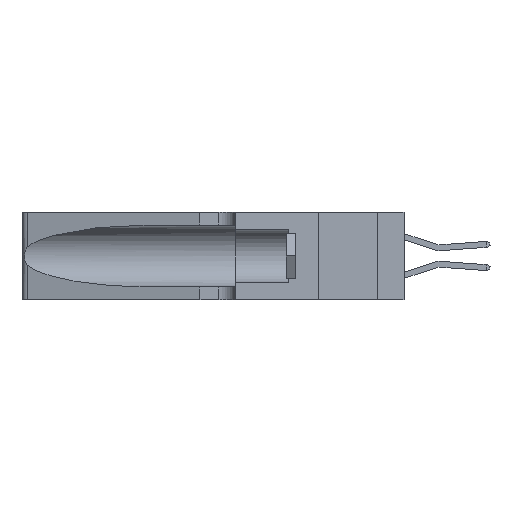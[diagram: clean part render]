
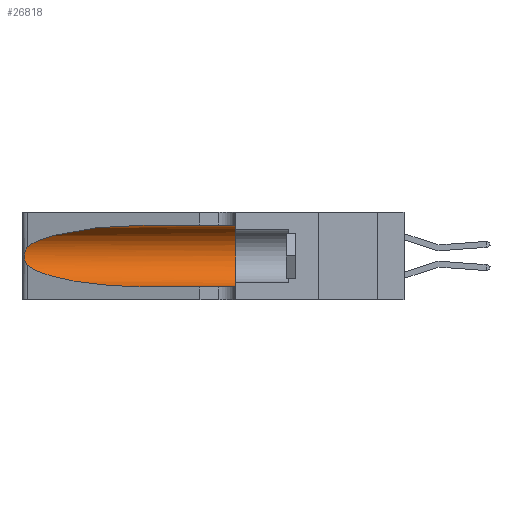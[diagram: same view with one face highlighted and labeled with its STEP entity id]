
A CAD part, left-side view. The second image highlights one B-rep face of the part: STEP entity #26818.
In plain terms, the highlighted cylindrical face has radius 3.308 mm (diameter 6.617 mm), a partial arc.
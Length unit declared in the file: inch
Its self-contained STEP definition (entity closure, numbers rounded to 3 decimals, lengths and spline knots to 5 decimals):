
#144 = CARTESIAN_POINT ( 'NONE',  ( 0.25856, 1.23593, 0.16098 ) ) ;
#509 = CIRCLE ( 'NONE', #16117, 0.13025 ) ;
#758 = CARTESIAN_POINT ( 'NONE',  ( 0.1305, 1.61858, 0.05475 ) ) ;
#2188 = EDGE_CURVE ( 'NONE', #5436, #7439, #509, .T. ) ;
#2195 = VERTEX_POINT ( 'NONE', #33431 ) ;
#3414 = CARTESIAN_POINT ( 'NONE',  ( 0.25639, 1.23186, 0.15144 ) ) ;
#3871 = CARTESIAN_POINT ( 'NONE',  ( 0.18966, 0.96281, 0.05475 ) ) ;
#3961 = CARTESIAN_POINT ( 'NONE',  ( 0.2373, 1.15595, 0.28018 ) ) ;
#5436 = VERTEX_POINT ( 'NONE', #6036 ) ;
#5816 = DIRECTION ( 'NONE',  ( 0., 0., -1. ) ) ;
#5820 = B_SPLINE_CURVE_WITH_KNOTS ( 'NONE', 3,
 ( #22735, #19509, #9816, #32449, #13088, #35671, #16386, #38870, #19641, #144, #22863, #3414, #26111, #6705 ),
 .UNSPECIFIED., .F., .F.,
 ( 4, 2, 2, 2, 2, 2, 4 ),
 ( 0., 0.00027, 0.00053, 0.00107, 0.0016, 0.00187, 0.00214 ),
 .UNSPECIFIED. ) ;
#6036 = CARTESIAN_POINT ( 'NONE',  ( 0.1305, 0.35, 0.31525 ) ) ;
#6705 = CARTESIAN_POINT ( 'NONE',  ( 0.25487, 1.22718, 0.14631 ) ) ;
#6892 = LINE ( 'NONE', #22864, #31703 ) ;
#7290 = CYLINDRICAL_SURFACE ( 'NONE', #20768, 0.13025 ) ;
#7439 = VERTEX_POINT ( 'NONE', #38332 ) ;
#9204 = DIRECTION ( 'NONE',  ( 0., -1., 0. ) ) ;
#9816 = CARTESIAN_POINT ( 'NONE',  ( 0.25639, 1.23184, 0.21858 ) ) ;
#10244 =( BOUNDED_CURVE ( )  B_SPLINE_CURVE ( 3, ( #26418, #36107, #3871, #26557 ),
 .UNSPECIFIED., .F., .T. ) 
 B_SPLINE_CURVE_WITH_KNOTS ( ( 4, 4 ),
 ( 3.44316, 4.71239 ),
 .UNSPECIFIED. ) 
 CURVE ( )  GEOMETRIC_REPRESENTATION_ITEM ( )  RATIONAL_B_SPLINE_CURVE ( ( 1., 0.87, 0.87, 1. ) ) 
 REPRESENTATION_ITEM ( '' )  );
#10946 = CARTESIAN_POINT ( 'NONE',  ( 0.1305, 0.35, 0.185 ) ) ;
#12479 = CARTESIAN_POINT ( 'NONE',  ( 0.1305, 1.61858, 0.185 ) ) ;
#12676 = EDGE_CURVE ( 'NONE', #41660, #5436, #6892, .T. ) ;
#13088 = CARTESIAN_POINT ( 'NONE',  ( 0.25854, 1.2359, 0.20912 ) ) ;
#13367 =( BOUNDED_CURVE ( )  B_SPLINE_CURVE ( 3, ( #32978, #36195, #3961, #26655 ),
 .UNSPECIFIED., .F., .F. ) 
 B_SPLINE_CURVE_WITH_KNOTS ( ( 4, 4 ),
 ( 1.5708, 2.84003 ),
 .UNSPECIFIED. ) 
 CURVE ( )  GEOMETRIC_REPRESENTATION_ITEM ( )  RATIONAL_B_SPLINE_CURVE ( ( 1., 0.87, 0.87, 1. ) ) 
 REPRESENTATION_ITEM ( '' )  );
#13708 = LINE ( 'NONE', #758, #36399 ) ;
#14234 = DIRECTION ( 'NONE',  ( 0., 0., 1. ) ) ;
#15229 = CARTESIAN_POINT ( 'NONE',  ( 0.1305, 0.72297, 0.05475 ) ) ;
#16117 = AXIS2_PLACEMENT_3D ( 'NONE', #10946, #33566, #14234 ) ;
#16257 = EDGE_CURVE ( 'NONE', #27546, #7439, #13708, .T. ) ;
#16386 = CARTESIAN_POINT ( 'NONE',  ( 0.26075, 1.23896, 0.19203 ) ) ;
#16870 = ORIENTED_EDGE ( 'NONE', *, *, #16257, .T. ) ;
#19509 = CARTESIAN_POINT ( 'NONE',  ( 0.25555, 1.22994, 0.2215 ) ) ;
#19641 = CARTESIAN_POINT ( 'NONE',  ( 0.26017, 1.23833, 0.17102 ) ) ;
#20768 = AXIS2_PLACEMENT_3D ( 'NONE', #12479, #9204, #5816 ) ;
#22572 = ORIENTED_EDGE ( 'NONE', *, *, #12676, .F. ) ;
#22735 = CARTESIAN_POINT ( 'NONE',  ( 0.25487, 1.22718, 0.22369 ) ) ;
#22863 = CARTESIAN_POINT ( 'NONE',  ( 0.25789, 1.23486, 0.15765 ) ) ;
#22864 = CARTESIAN_POINT ( 'NONE',  ( 0.1305, 1.61858, 0.31525 ) ) ;
#23547 = EDGE_CURVE ( 'NONE', #41660, #2195, #13367, .T. ) ;
#24517 = FACE_OUTER_BOUND ( 'NONE', #35271, .T. ) ;
#26111 = CARTESIAN_POINT ( 'NONE',  ( 0.25555, 1.22993, 0.14849 ) ) ;
#26113 = DIRECTION ( 'NONE',  ( 0., -1., 0. ) ) ;
#26264 = EDGE_CURVE ( 'NONE', #2195, #33446, #5820, .T. ) ;
#26311 = CARTESIAN_POINT ( 'NONE',  ( 0.1305, 0.72297, 0.31525 ) ) ;
#26418 = CARTESIAN_POINT ( 'NONE',  ( 0.25487, 1.22718, 0.14631 ) ) ;
#26557 = CARTESIAN_POINT ( 'NONE',  ( 0.1305, 0.72297, 0.05475 ) ) ;
#26572 = DIRECTION ( 'NONE',  ( 0., -1., 0. ) ) ;
#26655 = CARTESIAN_POINT ( 'NONE',  ( 0.25487, 1.22718, 0.22369 ) ) ;
#26818 = ADVANCED_FACE ( 'NONE', ( #24517 ), #7290, .F. ) ;
#27546 = VERTEX_POINT ( 'NONE', #15229 ) ;
#27749 = ORIENTED_EDGE ( 'NONE', *, *, #23547, .T. ) ;
#31703 = VECTOR ( 'NONE', #26113, 39.37008 ) ;
#32449 = CARTESIAN_POINT ( 'NONE',  ( 0.25787, 1.23484, 0.2124 ) ) ;
#32816 = CARTESIAN_POINT ( 'NONE',  ( 0.25487, 1.22718, 0.14631 ) ) ;
#32978 = CARTESIAN_POINT ( 'NONE',  ( 0.1305, 0.72297, 0.31525 ) ) ;
#33273 = ORIENTED_EDGE ( 'NONE', *, *, #40409, .T. ) ;
#33431 = CARTESIAN_POINT ( 'NONE',  ( 0.25487, 1.22718, 0.22369 ) ) ;
#33446 = VERTEX_POINT ( 'NONE', #32816 ) ;
#33566 = DIRECTION ( 'NONE',  ( 0., 1., 0. ) ) ;
#35271 = EDGE_LOOP ( 'NONE', ( #27749, #39455, #33273, #16870, #36765, #22572 ) ) ;
#35671 = CARTESIAN_POINT ( 'NONE',  ( 0.26018, 1.23835, 0.19895 ) ) ;
#36107 = CARTESIAN_POINT ( 'NONE',  ( 0.2373, 1.15595, 0.08982 ) ) ;
#36195 = CARTESIAN_POINT ( 'NONE',  ( 0.18966, 0.96281, 0.31525 ) ) ;
#36399 = VECTOR ( 'NONE', #26572, 39.37008 ) ;
#36765 = ORIENTED_EDGE ( 'NONE', *, *, #2188, .F. ) ;
#38332 = CARTESIAN_POINT ( 'NONE',  ( 0.1305, 0.35, 0.05475 ) ) ;
#38870 = CARTESIAN_POINT ( 'NONE',  ( 0.26075, 1.23896, 0.178 ) ) ;
#39455 = ORIENTED_EDGE ( 'NONE', *, *, #26264, .T. ) ;
#40409 = EDGE_CURVE ( 'NONE', #33446, #27546, #10244, .T. ) ;
#41660 = VERTEX_POINT ( 'NONE', #26311 ) ;
